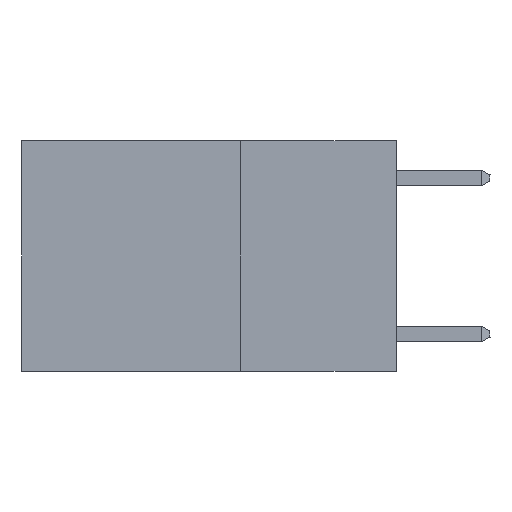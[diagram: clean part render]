
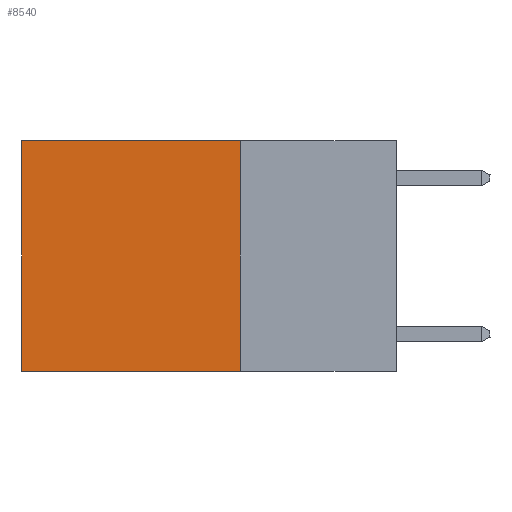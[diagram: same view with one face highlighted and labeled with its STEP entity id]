
A CAD part, left-side view. The second image highlights one B-rep face of the part: STEP entity #8540.
In plain terms, the highlighted planar face has unit normal (-1, 0, 0).
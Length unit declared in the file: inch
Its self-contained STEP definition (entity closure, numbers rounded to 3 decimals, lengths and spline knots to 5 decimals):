
#171 = LINE ( 'NONE', #2118, #9469 ) ;
#200 = AXIS2_PLACEMENT_3D ( 'NONE', #3160, #10891, #1467 ) ;
#707 = ORIENTED_EDGE ( 'NONE', *, *, #6460, .T. ) ;
#878 = CARTESIAN_POINT ( 'NONE',  ( 0.2625, 0.6, 0. ) ) ;
#1024 = CARTESIAN_POINT ( 'NONE',  ( 0.2625, 0.25, 0. ) ) ;
#1158 = EDGE_CURVE ( 'NONE', #4564, #7633, #4297, .T. ) ;
#1467 = DIRECTION ( 'NONE',  ( 0., 0., -1. ) ) ;
#1487 = DIRECTION ( 'NONE',  ( 0., 0., -1. ) ) ;
#1540 = LINE ( 'NONE', #5927, #7000 ) ;
#2118 = CARTESIAN_POINT ( 'NONE',  ( 0.2625, 0.25, -0.37 ) ) ;
#2160 = FACE_OUTER_BOUND ( 'NONE', #11011, .T. ) ;
#2841 = ORIENTED_EDGE ( 'NONE', *, *, #3132, .T. ) ;
#3132 = EDGE_CURVE ( 'NONE', #8754, #7350, #1540, .T. ) ;
#3160 = CARTESIAN_POINT ( 'NONE',  ( 0.2625, 0.25, 0. ) ) ;
#3452 = CARTESIAN_POINT ( 'NONE',  ( 0.2625, 0.25, 0. ) ) ;
#3674 = CARTESIAN_POINT ( 'NONE',  ( 0.2625, 0.25, 0. ) ) ;
#3771 = CARTESIAN_POINT ( 'NONE',  ( 0.2625, 0.6, -0.37 ) ) ;
#4297 = LINE ( 'NONE', #3452, #6292 ) ;
#4564 = VERTEX_POINT ( 'NONE', #3674 ) ;
#5300 = DIRECTION ( 'NONE',  ( 0., 0., -1. ) ) ;
#5745 = PLANE ( 'NONE',  #200 ) ;
#5927 = CARTESIAN_POINT ( 'NONE',  ( 0.2625, 0.6, 0. ) ) ;
#6292 = VECTOR ( 'NONE', #5300, 39.37008 ) ;
#6414 = ORIENTED_EDGE ( 'NONE', *, *, #6491, .F. ) ;
#6460 = EDGE_CURVE ( 'NONE', #4564, #8754, #7091, .T. ) ;
#6491 = EDGE_CURVE ( 'NONE', #7633, #7350, #171, .T. ) ;
#7000 = VECTOR ( 'NONE', #1487, 39.37008 ) ;
#7091 = LINE ( 'NONE', #1024, #9098 ) ;
#7350 = VERTEX_POINT ( 'NONE', #3771 ) ;
#7633 = VERTEX_POINT ( 'NONE', #8284 ) ;
#7954 = ORIENTED_EDGE ( 'NONE', *, *, #1158, .F. ) ;
#8284 = CARTESIAN_POINT ( 'NONE',  ( 0.2625, 0.25, -0.37 ) ) ;
#8357 = DIRECTION ( 'NONE',  ( 0., 1., 0. ) ) ;
#8540 = ADVANCED_FACE ( 'NONE', ( #2160 ), #5745, .F. ) ;
#8754 = VERTEX_POINT ( 'NONE', #878 ) ;
#9098 = VECTOR ( 'NONE', #9937, 39.37008 ) ;
#9469 = VECTOR ( 'NONE', #8357, 39.37008 ) ;
#9937 = DIRECTION ( 'NONE',  ( 0., 1., 0. ) ) ;
#10891 = DIRECTION ( 'NONE',  ( 1., 0., 0. ) ) ;
#11011 = EDGE_LOOP ( 'NONE', ( #2841, #6414, #7954, #707 ) ) ;
